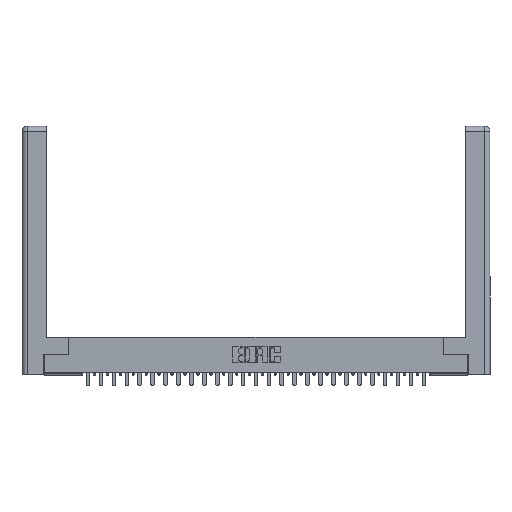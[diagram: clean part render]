
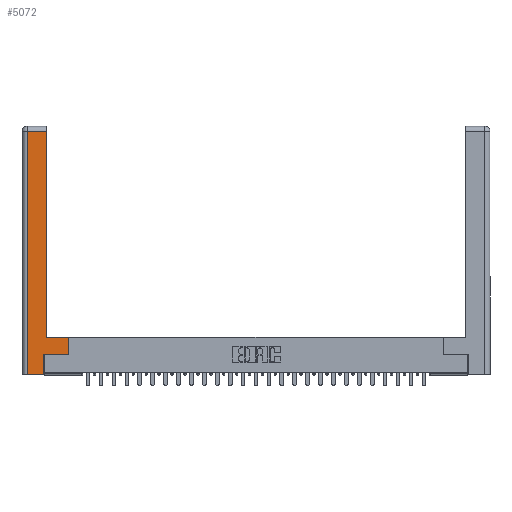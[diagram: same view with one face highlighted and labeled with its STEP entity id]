
A CAD part, top view. The second image highlights one B-rep face of the part: STEP entity #5072.
In plain terms, the highlighted planar face has unit normal (0, 0, 1).
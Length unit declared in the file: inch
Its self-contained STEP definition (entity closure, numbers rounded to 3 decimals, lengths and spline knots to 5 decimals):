
#904 = VERTEX_POINT ( 'NONE', #19988 ) ;
#1042 = VERTEX_POINT ( 'NONE', #32098 ) ;
#1114 = AXIS2_PLACEMENT_3D ( 'NONE', #10850, #28519, #13463 ) ;
#1138 = VERTEX_POINT ( 'NONE', #1933 ) ;
#1933 = CARTESIAN_POINT ( 'NONE',  ( 0.565, 0.45, 0. ) ) ;
#2960 = VECTOR ( 'NONE', #3818, 39.37008 ) ;
#3818 = DIRECTION ( 'NONE',  ( 0., 1., 0. ) ) ;
#4237 = LINE ( 'NONE', #9447, #15575 ) ;
#4288 = DIRECTION ( 'NONE',  ( 0., 1., 0. ) ) ;
#4537 = VERTEX_POINT ( 'NONE', #31726 ) ;
#5072 = ADVANCED_FACE ( 'NONE', ( #18161 ), #31466, .F. ) ;
#5095 = EDGE_CURVE ( 'NONE', #25174, #904, #13725, .T. ) ;
#5304 = DIRECTION ( 'NONE',  ( -1., 0., 0. ) ) ;
#5775 = VERTEX_POINT ( 'NONE', #18112 ) ;
#6093 = DIRECTION ( 'NONE',  ( 1., 0., 0. ) ) ;
#6597 = CARTESIAN_POINT ( 'NONE',  ( 0.0615, 0., 0. ) ) ;
#7189 = EDGE_CURVE ( 'NONE', #5775, #14675, #15785, .T. ) ;
#7672 = DIRECTION ( 'NONE',  ( 1., 0., 0. ) ) ;
#7713 = VECTOR ( 'NONE', #4288, 39.37008 ) ;
#9447 = CARTESIAN_POINT ( 'NONE',  ( 0.0615, 0., 0. ) ) ;
#9562 = DIRECTION ( 'NONE',  ( 0., -1., 0. ) ) ;
#9957 = EDGE_LOOP ( 'NONE', ( #14197, #20889, #29812, #24327, #18208, #32513, #23582, #16579 ) ) ;
#10606 = CARTESIAN_POINT ( 'NONE',  ( 0.265, 0.245, 0. ) ) ;
#10826 = EDGE_CURVE ( 'NONE', #4537, #25174, #13965, .T. ) ;
#10850 = CARTESIAN_POINT ( 'NONE',  ( 0., 0., 0. ) ) ;
#10968 = EDGE_CURVE ( 'NONE', #904, #22941, #4237, .T. ) ;
#13221 = VECTOR ( 'NONE', #7672, 39.37008 ) ;
#13463 = DIRECTION ( 'NONE',  ( -1., 0., 0. ) ) ;
#13725 = LINE ( 'NONE', #21028, #19407 ) ;
#13804 = EDGE_CURVE ( 'NONE', #1042, #1138, #23536, .T. ) ;
#13965 = LINE ( 'NONE', #25290, #16821 ) ;
#14171 = DIRECTION ( 'NONE',  ( -1., 0., 0. ) ) ;
#14197 = ORIENTED_EDGE ( 'NONE', *, *, #10826, .T. ) ;
#14675 = VERTEX_POINT ( 'NONE', #10606 ) ;
#15479 = CARTESIAN_POINT ( 'NONE',  ( 0.265, 0., 0. ) ) ;
#15575 = VECTOR ( 'NONE', #9562, 39.37008 ) ;
#15785 = LINE ( 'NONE', #27698, #7713 ) ;
#16579 = ORIENTED_EDGE ( 'NONE', *, *, #23072, .T. ) ;
#16821 = VECTOR ( 'NONE', #30644, 39.37008 ) ;
#17217 = VECTOR ( 'NONE', #6093, 39.37008 ) ;
#17633 = LINE ( 'NONE', #31932, #17217 ) ;
#18112 = CARTESIAN_POINT ( 'NONE',  ( 0.265, 0., 0. ) ) ;
#18161 = FACE_OUTER_BOUND ( 'NONE', #9957, .T. ) ;
#18208 = ORIENTED_EDGE ( 'NONE', *, *, #7189, .T. ) ;
#19407 = VECTOR ( 'NONE', #5304, 39.37008 ) ;
#19988 = CARTESIAN_POINT ( 'NONE',  ( 0.0615, 2.94, 0. ) ) ;
#20889 = ORIENTED_EDGE ( 'NONE', *, *, #5095, .T. ) ;
#21028 = CARTESIAN_POINT ( 'NONE',  ( 0.0615, 2.94, 0. ) ) ;
#21263 = EDGE_CURVE ( 'NONE', #14675, #1042, #17633, .T. ) ;
#22941 = VERTEX_POINT ( 'NONE', #6597 ) ;
#22970 = VECTOR ( 'NONE', #14171, 39.37008 ) ;
#23072 = EDGE_CURVE ( 'NONE', #1138, #4537, #29924, .T. ) ;
#23536 = LINE ( 'NONE', #26943, #2960 ) ;
#23582 = ORIENTED_EDGE ( 'NONE', *, *, #13804, .T. ) ;
#24327 = ORIENTED_EDGE ( 'NONE', *, *, #25197, .T. ) ;
#25174 = VERTEX_POINT ( 'NONE', #28370 ) ;
#25197 = EDGE_CURVE ( 'NONE', #22941, #5775, #26985, .T. ) ;
#25290 = CARTESIAN_POINT ( 'NONE',  ( 0.295, 3., 0. ) ) ;
#26943 = CARTESIAN_POINT ( 'NONE',  ( 0.565, 0.45, 0. ) ) ;
#26985 = LINE ( 'NONE', #15479, #13221 ) ;
#27698 = CARTESIAN_POINT ( 'NONE',  ( 0.265, 0.245, 0. ) ) ;
#28370 = CARTESIAN_POINT ( 'NONE',  ( 0.295, 2.94, 0. ) ) ;
#28519 = DIRECTION ( 'NONE',  ( 0., 0., -1. ) ) ;
#29203 = CARTESIAN_POINT ( 'NONE',  ( 0.295, 0.45, 0. ) ) ;
#29812 = ORIENTED_EDGE ( 'NONE', *, *, #10968, .T. ) ;
#29924 = LINE ( 'NONE', #29203, #22970 ) ;
#30644 = DIRECTION ( 'NONE',  ( 0., 1., 0. ) ) ;
#31466 = PLANE ( 'NONE',  #1114 ) ;
#31726 = CARTESIAN_POINT ( 'NONE',  ( 0.295, 0.45, 0. ) ) ;
#31932 = CARTESIAN_POINT ( 'NONE',  ( 0.565, 0.245, 0. ) ) ;
#32098 = CARTESIAN_POINT ( 'NONE',  ( 0.565, 0.245, 0. ) ) ;
#32513 = ORIENTED_EDGE ( 'NONE', *, *, #21263, .T. ) ;
